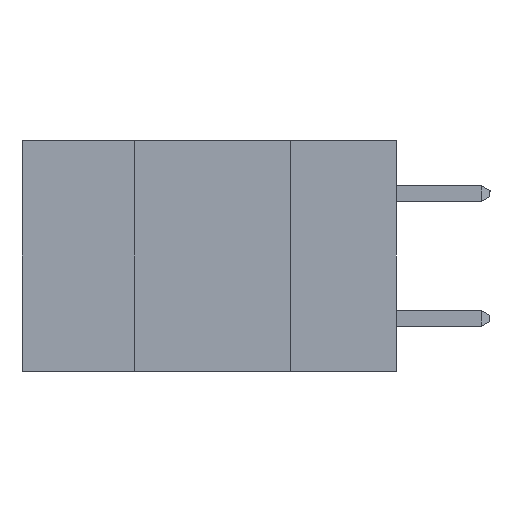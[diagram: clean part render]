
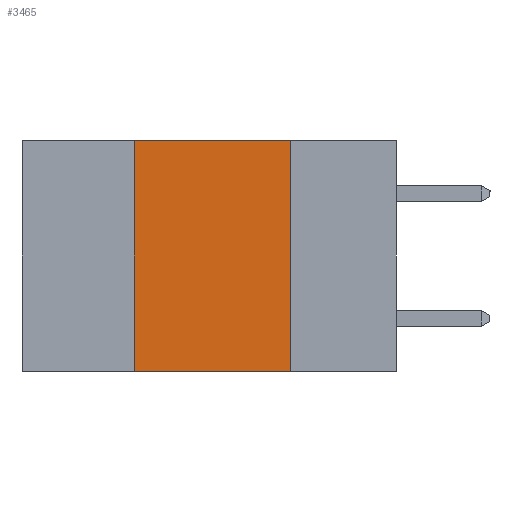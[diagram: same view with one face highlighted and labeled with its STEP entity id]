
A CAD part, left-side view. The second image highlights one B-rep face of the part: STEP entity #3465.
In plain terms, the highlighted planar face has unit normal (-1, 0, 0).
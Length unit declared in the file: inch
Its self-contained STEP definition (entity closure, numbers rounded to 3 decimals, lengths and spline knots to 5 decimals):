
#293 = EDGE_CURVE ( 'NONE', #1416, #6957, #4719, .T. ) ;
#677 = DIRECTION ( 'NONE',  ( 1., 0., 0. ) ) ;
#916 = VECTOR ( 'NONE', #9956, 39.37008 ) ;
#1416 = VERTEX_POINT ( 'NONE', #9423 ) ;
#2241 = CARTESIAN_POINT ( 'NONE',  ( 0., 0.6, -0.37 ) ) ;
#2521 = DIRECTION ( 'NONE',  ( 0., -1., 0. ) ) ;
#3363 = EDGE_CURVE ( 'NONE', #1416, #8829, #9759, .T. ) ;
#3465 = ADVANCED_FACE ( 'NONE', ( #8928 ), #6005, .F. ) ;
#3816 = DIRECTION ( 'NONE',  ( 0., 0., -1. ) ) ;
#4544 = CARTESIAN_POINT ( 'NONE',  ( 0., 0.6, 0. ) ) ;
#4719 = LINE ( 'NONE', #4778, #12117 ) ;
#4778 = CARTESIAN_POINT ( 'NONE',  ( 0., 0.42, -0.37 ) ) ;
#5426 = LINE ( 'NONE', #4544, #12519 ) ;
#5478 = EDGE_CURVE ( 'NONE', #10556, #8829, #5867, .T. ) ;
#5570 = DIRECTION ( 'NONE',  ( 0., -1., 0. ) ) ;
#5867 = LINE ( 'NONE', #13019, #916 ) ;
#6005 = PLANE ( 'NONE',  #7907 ) ;
#6087 = DIRECTION ( 'NONE',  ( 0., 0., 1. ) ) ;
#6957 = VERTEX_POINT ( 'NONE', #7912 ) ;
#7028 = CARTESIAN_POINT ( 'NONE',  ( 0., 0.17, -0.37 ) ) ;
#7907 = AXIS2_PLACEMENT_3D ( 'NONE', #9953, #677, #3816 ) ;
#7912 = CARTESIAN_POINT ( 'NONE',  ( 0., 0.42, 0. ) ) ;
#8829 = VERTEX_POINT ( 'NONE', #7028 ) ;
#8928 = FACE_OUTER_BOUND ( 'NONE', #11241, .T. ) ;
#8930 = EDGE_CURVE ( 'NONE', #6957, #10556, #5426, .T. ) ;
#8957 = ORIENTED_EDGE ( 'NONE', *, *, #8930, .F. ) ;
#9423 = CARTESIAN_POINT ( 'NONE',  ( 0., 0.42, -0.37 ) ) ;
#9759 = LINE ( 'NONE', #2241, #10550 ) ;
#9953 = CARTESIAN_POINT ( 'NONE',  ( 0., 0.6, 0. ) ) ;
#9956 = DIRECTION ( 'NONE',  ( 0., 0., -1. ) ) ;
#9994 = CARTESIAN_POINT ( 'NONE',  ( 0., 0.17, 0. ) ) ;
#10020 = ORIENTED_EDGE ( 'NONE', *, *, #5478, .F. ) ;
#10231 = ORIENTED_EDGE ( 'NONE', *, *, #3363, .T. ) ;
#10550 = VECTOR ( 'NONE', #2521, 39.37008 ) ;
#10556 = VERTEX_POINT ( 'NONE', #9994 ) ;
#11140 = ORIENTED_EDGE ( 'NONE', *, *, #293, .F. ) ;
#11241 = EDGE_LOOP ( 'NONE', ( #10020, #8957, #11140, #10231 ) ) ;
#12117 = VECTOR ( 'NONE', #6087, 39.37008 ) ;
#12519 = VECTOR ( 'NONE', #5570, 39.37008 ) ;
#13019 = CARTESIAN_POINT ( 'NONE',  ( 0., 0.17, -0.37 ) ) ;
